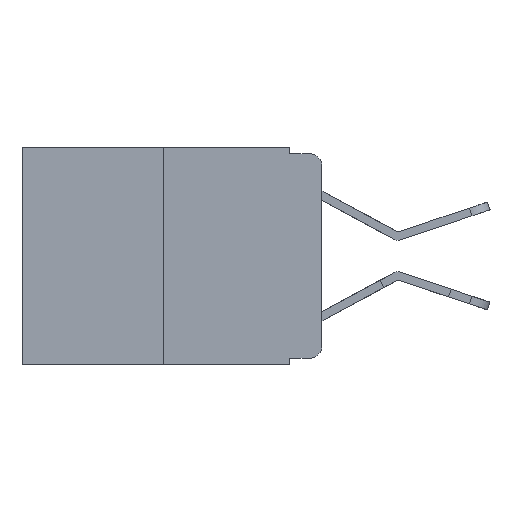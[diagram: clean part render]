
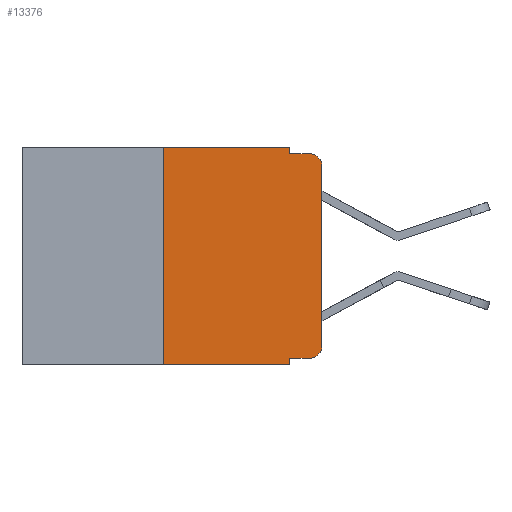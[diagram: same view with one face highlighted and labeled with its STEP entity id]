
A CAD part, left-side view. The second image highlights one B-rep face of the part: STEP entity #13376.
In plain terms, the highlighted planar face has unit normal (-1, 0, 0).
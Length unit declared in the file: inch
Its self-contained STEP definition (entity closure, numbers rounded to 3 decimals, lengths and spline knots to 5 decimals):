
#90 = VECTOR ( 'NONE', #11641, 39.37008 ) ;
#561 = DIRECTION ( 'NONE',  ( 0., 0., 1. ) ) ;
#830 = LINE ( 'NONE', #21411, #16387 ) ;
#860 = DIRECTION ( 'NONE',  ( 0., 0., -1. ) ) ;
#1023 = VERTEX_POINT ( 'NONE', #20550 ) ;
#1119 = DIRECTION ( 'NONE',  ( 0., 0., -1. ) ) ;
#1436 = DIRECTION ( 'NONE',  ( 0., 0., -1. ) ) ;
#1583 = DIRECTION ( 'NONE',  ( 0., -1., 0. ) ) ;
#1867 = DIRECTION ( 'NONE',  ( 0., 0., -1. ) ) ;
#2036 = ORIENTED_EDGE ( 'NONE', *, *, #17071, .T. ) ;
#2514 = CARTESIAN_POINT ( 'NONE',  ( 0., 0.25, -0.343 ) ) ;
#2521 = VERTEX_POINT ( 'NONE', #2514 ) ;
#3278 = VECTOR ( 'NONE', #9961, 39.37008 ) ;
#3337 = ORIENTED_EDGE ( 'NONE', *, *, #18102, .F. ) ;
#4139 = CARTESIAN_POINT ( 'NONE',  ( 0., 0.02, -0.333 ) ) ;
#5041 = ORIENTED_EDGE ( 'NONE', *, *, #6852, .F. ) ;
#5232 = VECTOR ( 'NONE', #21034, 39.37008 ) ;
#5569 = DIRECTION ( 'NONE',  ( 0., 0., 1. ) ) ;
#6852 = EDGE_CURVE ( 'NONE', #1023, #18766, #14031, .T. ) ;
#7096 = CARTESIAN_POINT ( 'NONE',  ( 0., 0.473, -0.343 ) ) ;
#7671 = CARTESIAN_POINT ( 'NONE',  ( 0., 0.051, -0.333 ) ) ;
#8738 = EDGE_CURVE ( 'NONE', #8873, #9482, #16095, .T. ) ;
#8764 = CARTESIAN_POINT ( 'NONE',  ( 0., 0.25, 0. ) ) ;
#8873 = VERTEX_POINT ( 'NONE', #16161 ) ;
#8896 = CARTESIAN_POINT ( 'NONE',  ( 0., 0.051, 0. ) ) ;
#9273 = CARTESIAN_POINT ( 'NONE',  ( 0., 0., -0.03 ) ) ;
#9445 = DIRECTION ( 'NONE',  ( 0., -1., 0. ) ) ;
#9482 = VERTEX_POINT ( 'NONE', #4139 ) ;
#9598 = CARTESIAN_POINT ( 'NONE',  ( 0., 0.051, 0. ) ) ;
#9740 = VECTOR ( 'NONE', #860, 39.37008 ) ;
#9930 = VECTOR ( 'NONE', #5569, 39.37008 ) ;
#9961 = DIRECTION ( 'NONE',  ( 0., -1., 0. ) ) ;
#10786 = VECTOR ( 'NONE', #1583, 39.37008 ) ;
#11029 = LINE ( 'NONE', #9598, #90 ) ;
#11089 = EDGE_CURVE ( 'NONE', #15986, #15317, #18253, .T. ) ;
#11197 = CARTESIAN_POINT ( 'NONE',  ( 0., 0.051, -0.343 ) ) ;
#11235 = CARTESIAN_POINT ( 'NONE',  ( 0., 0.02, -0.01 ) ) ;
#11625 = PLANE ( 'NONE',  #25746 ) ;
#11641 = DIRECTION ( 'NONE',  ( 0., 0., -1. ) ) ;
#11866 = LINE ( 'NONE', #7096, #5232 ) ;
#12003 = CARTESIAN_POINT ( 'NONE',  ( 0., 0.473, 0. ) ) ;
#12099 = VECTOR ( 'NONE', #561, 39.37008 ) ;
#13084 = CARTESIAN_POINT ( 'NONE',  ( 0., 0.051, 0. ) ) ;
#13126 = ORIENTED_EDGE ( 'NONE', *, *, #20735, .F. ) ;
#13316 = DIRECTION ( 'NONE',  ( -1., 0., 0. ) ) ;
#13376 = ADVANCED_FACE ( 'NONE', ( #22684 ), #11625, .F. ) ;
#13612 = DIRECTION ( 'NONE',  ( 1., 0., 0. ) ) ;
#13775 = AXIS2_PLACEMENT_3D ( 'NONE', #25749, #14016, #1867 ) ;
#14016 = DIRECTION ( 'NONE',  ( -1., 0., 0. ) ) ;
#14031 = LINE ( 'NONE', #12003, #3278 ) ;
#14125 = EDGE_CURVE ( 'NONE', #9482, #14809, #22960, .T. ) ;
#14164 = ORIENTED_EDGE ( 'NONE', *, *, #19904, .F. ) ;
#14617 = EDGE_CURVE ( 'NONE', #14809, #15986, #25040, .T. ) ;
#14809 = VERTEX_POINT ( 'NONE', #19498 ) ;
#15317 = VERTEX_POINT ( 'NONE', #11235 ) ;
#15557 = CARTESIAN_POINT ( 'NONE',  ( 0., 0., 0. ) ) ;
#15735 = AXIS2_PLACEMENT_3D ( 'NONE', #25059, #13316, #1119 ) ;
#15986 = VERTEX_POINT ( 'NONE', #9273 ) ;
#16095 = LINE ( 'NONE', #7671, #10786 ) ;
#16161 = CARTESIAN_POINT ( 'NONE',  ( 0., 0.051, -0.333 ) ) ;
#16168 = ORIENTED_EDGE ( 'NONE', *, *, #21220, .F. ) ;
#16387 = VECTOR ( 'NONE', #9445, 39.37008 ) ;
#17071 = EDGE_CURVE ( 'NONE', #2521, #18856, #11866, .T. ) ;
#17381 = LINE ( 'NONE', #8764, #12099 ) ;
#17451 = ORIENTED_EDGE ( 'NONE', *, *, #8738, .T. ) ;
#17525 = CARTESIAN_POINT ( 'NONE',  ( 0., 0.473, 0. ) ) ;
#18102 = EDGE_CURVE ( 'NONE', #2521, #1023, #17381, .T. ) ;
#18253 = CIRCLE ( 'NONE', #15735, 0.02 ) ;
#18766 = VERTEX_POINT ( 'NONE', #8896 ) ;
#18856 = VERTEX_POINT ( 'NONE', #11197 ) ;
#19129 = CARTESIAN_POINT ( 'NONE',  ( 0., 0.051, -0.01 ) ) ;
#19498 = CARTESIAN_POINT ( 'NONE',  ( 0., 0., -0.313 ) ) ;
#19904 = EDGE_CURVE ( 'NONE', #22367, #15317, #830, .T. ) ;
#20316 = LINE ( 'NONE', #13084, #9740 ) ;
#20550 = CARTESIAN_POINT ( 'NONE',  ( 0., 0.25, 0. ) ) ;
#20735 = EDGE_CURVE ( 'NONE', #8873, #18856, #11029, .T. ) ;
#21034 = DIRECTION ( 'NONE',  ( 0., -1., 0. ) ) ;
#21220 = EDGE_CURVE ( 'NONE', #18766, #22367, #20316, .T. ) ;
#21230 = ORIENTED_EDGE ( 'NONE', *, *, #14617, .T. ) ;
#21411 = CARTESIAN_POINT ( 'NONE',  ( 0., 0.051, -0.01 ) ) ;
#22367 = VERTEX_POINT ( 'NONE', #19129 ) ;
#22684 = FACE_OUTER_BOUND ( 'NONE', #23236, .T. ) ;
#22960 = CIRCLE ( 'NONE', #13775, 0.02 ) ;
#23003 = ORIENTED_EDGE ( 'NONE', *, *, #14125, .T. ) ;
#23236 = EDGE_LOOP ( 'NONE', ( #21230, #25693, #14164, #16168, #5041, #3337, #2036, #13126, #17451, #23003 ) ) ;
#25040 = LINE ( 'NONE', #15557, #9930 ) ;
#25059 = CARTESIAN_POINT ( 'NONE',  ( 0., 0.02, -0.03 ) ) ;
#25693 = ORIENTED_EDGE ( 'NONE', *, *, #11089, .T. ) ;
#25746 = AXIS2_PLACEMENT_3D ( 'NONE', #17525, #13612, #1436 ) ;
#25749 = CARTESIAN_POINT ( 'NONE',  ( 0., 0.02, -0.313 ) ) ;
